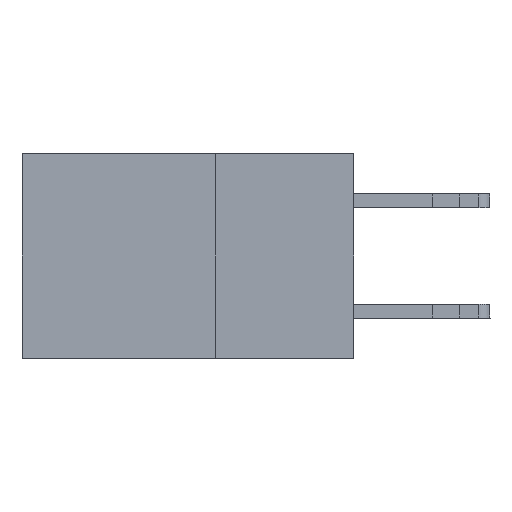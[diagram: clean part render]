
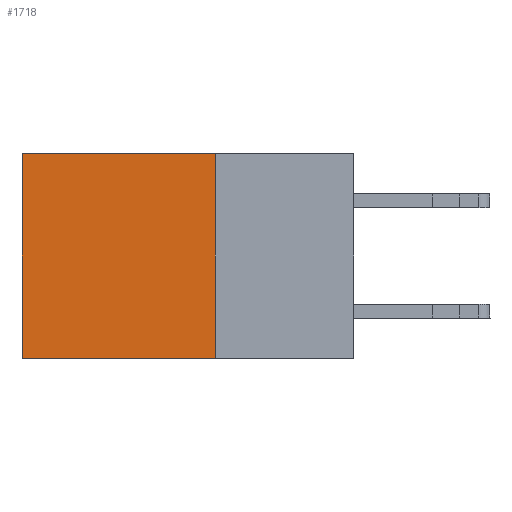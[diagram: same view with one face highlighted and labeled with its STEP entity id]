
A CAD part, left-side view. The second image highlights one B-rep face of the part: STEP entity #1718.
In plain terms, the highlighted planar face has unit normal (-1, 0, 0).
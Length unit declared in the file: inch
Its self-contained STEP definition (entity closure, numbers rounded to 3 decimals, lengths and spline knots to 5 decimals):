
#925 = LINE ( 'NONE', #3862, #12836 ) ;
#1185 = CARTESIAN_POINT ( 'NONE',  ( 0.2875, 0.25, 0. ) ) ;
#1437 = VECTOR ( 'NONE', #18011, 39.37008 ) ;
#1718 = ADVANCED_FACE ( 'NONE', ( #8500 ), #16020, .F. ) ;
#2056 = CARTESIAN_POINT ( 'NONE',  ( 0.2875, 0.25, -0.37 ) ) ;
#2906 = VERTEX_POINT ( 'NONE', #14697 ) ;
#2958 = EDGE_LOOP ( 'NONE', ( #9716, #4625, #3000, #11599 ) ) ;
#3000 = ORIENTED_EDGE ( 'NONE', *, *, #19838, .F. ) ;
#3235 = LINE ( 'NONE', #8554, #18968 ) ;
#3269 = EDGE_CURVE ( 'NONE', #2906, #14682, #3235, .T. ) ;
#3590 = CARTESIAN_POINT ( 'NONE',  ( 0.2875, 0.6, -0.37 ) ) ;
#3709 = DIRECTION ( 'NONE',  ( 0., 1., 0. ) ) ;
#3862 = CARTESIAN_POINT ( 'NONE',  ( 0.2875, 0.25, 0. ) ) ;
#4014 = CARTESIAN_POINT ( 'NONE',  ( 0.2875, 0.25, 0. ) ) ;
#4625 = ORIENTED_EDGE ( 'NONE', *, *, #6105, .F. ) ;
#5124 = LINE ( 'NONE', #1185, #1437 ) ;
#5242 = CARTESIAN_POINT ( 'NONE',  ( 0.2875, 0.25, -0.37 ) ) ;
#5511 = VERTEX_POINT ( 'NONE', #4014 ) ;
#5909 = DIRECTION ( 'NONE',  ( 0., 0., -1. ) ) ;
#6105 = EDGE_CURVE ( 'NONE', #12724, #14682, #14888, .T. ) ;
#8500 = FACE_OUTER_BOUND ( 'NONE', #2958, .T. ) ;
#8554 = CARTESIAN_POINT ( 'NONE',  ( 0.2875, 0.6, 0. ) ) ;
#9716 = ORIENTED_EDGE ( 'NONE', *, *, #3269, .T. ) ;
#10060 = DIRECTION ( 'NONE',  ( 0., 0., -1. ) ) ;
#10857 = VECTOR ( 'NONE', #3709, 39.37008 ) ;
#11599 = ORIENTED_EDGE ( 'NONE', *, *, #12361, .T. ) ;
#12361 = EDGE_CURVE ( 'NONE', #5511, #2906, #5124, .T. ) ;
#12724 = VERTEX_POINT ( 'NONE', #5242 ) ;
#12836 = VECTOR ( 'NONE', #10060, 39.37008 ) ;
#14682 = VERTEX_POINT ( 'NONE', #3590 ) ;
#14697 = CARTESIAN_POINT ( 'NONE',  ( 0.2875, 0.6, 0. ) ) ;
#14888 = LINE ( 'NONE', #2056, #10857 ) ;
#15562 = CARTESIAN_POINT ( 'NONE',  ( 0.2875, 0.25, 0. ) ) ;
#15690 = DIRECTION ( 'NONE',  ( 1., 0., 0. ) ) ;
#15849 = AXIS2_PLACEMENT_3D ( 'NONE', #15562, #15690, #15872 ) ;
#15872 = DIRECTION ( 'NONE',  ( 0., 0., -1. ) ) ;
#16020 = PLANE ( 'NONE',  #15849 ) ;
#18011 = DIRECTION ( 'NONE',  ( 0., 1., 0. ) ) ;
#18968 = VECTOR ( 'NONE', #5909, 39.37008 ) ;
#19838 = EDGE_CURVE ( 'NONE', #5511, #12724, #925, .T. ) ;
